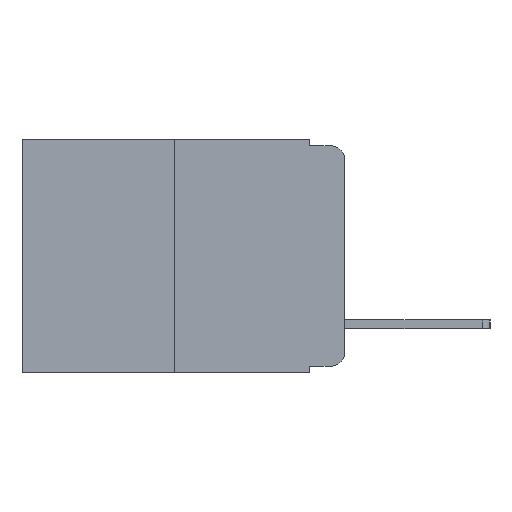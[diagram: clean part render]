
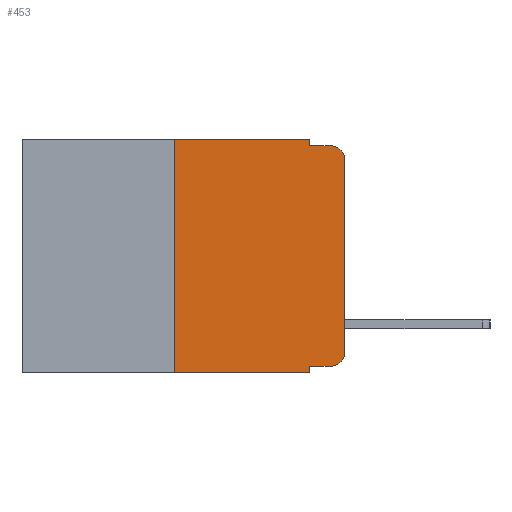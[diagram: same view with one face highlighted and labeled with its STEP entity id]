
A CAD part, left-side view. The second image highlights one B-rep face of the part: STEP entity #453.
In plain terms, the highlighted planar face has unit normal (-1, 0, 0).
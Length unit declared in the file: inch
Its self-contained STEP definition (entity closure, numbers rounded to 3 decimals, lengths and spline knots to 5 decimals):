
#366 = DIRECTION ( 'NONE',  ( 0., 0., 1. ) ) ;
#453 = ADVANCED_FACE ( 'NONE', ( #6808 ), #9087, .F. ) ;
#992 = CARTESIAN_POINT ( 'NONE',  ( 0., 0.25, 0. ) ) ;
#1239 = VERTEX_POINT ( 'NONE', #10865 ) ;
#1423 = DIRECTION ( 'NONE',  ( 0., -1., 0. ) ) ;
#1440 = CARTESIAN_POINT ( 'NONE',  ( 0., 0.051, 0. ) ) ;
#1443 = CARTESIAN_POINT ( 'NONE',  ( 0., 0., 0. ) ) ;
#1495 = VERTEX_POINT ( 'NONE', #3491 ) ;
#1644 = VECTOR ( 'NONE', #8561, 39.37008 ) ;
#1826 = CARTESIAN_POINT ( 'NONE',  ( 0., 0.051, -0.333 ) ) ;
#2103 = VERTEX_POINT ( 'NONE', #5677 ) ;
#2142 = VECTOR ( 'NONE', #11102, 39.37008 ) ;
#2264 = CARTESIAN_POINT ( 'NONE',  ( 0., 0.051, -0.01 ) ) ;
#2423 = VECTOR ( 'NONE', #1423, 39.37008 ) ;
#2447 = DIRECTION ( 'NONE',  ( 0., 0., -1. ) ) ;
#2634 = CARTESIAN_POINT ( 'NONE',  ( 0., 0.02, -0.333 ) ) ;
#2748 = AXIS2_PLACEMENT_3D ( 'NONE', #5929, #4686, #7265 ) ;
#3491 = CARTESIAN_POINT ( 'NONE',  ( 0., 0.051, -0.333 ) ) ;
#3553 = ORIENTED_EDGE ( 'NONE', *, *, #5797, .T. ) ;
#3752 = ORIENTED_EDGE ( 'NONE', *, *, #7470, .T. ) ;
#3794 = EDGE_CURVE ( 'NONE', #7345, #9619, #9673, .T. ) ;
#4267 = EDGE_CURVE ( 'NONE', #9619, #1239, #7231, .T. ) ;
#4373 = LINE ( 'NONE', #9382, #1644 ) ;
#4440 = EDGE_LOOP ( 'NONE', ( #3553, #3752, #4926, #5166, #5192, #5324, #5936, #6042, #6184, #6228 ) ) ;
#4561 = CARTESIAN_POINT ( 'NONE',  ( 0., 0.25, 0. ) ) ;
#4566 = DIRECTION ( 'NONE',  ( -1., 0., 0. ) ) ;
#4616 = CARTESIAN_POINT ( 'NONE',  ( 0., 0.02, -0.313 ) ) ;
#4645 = CIRCLE ( 'NONE', #5141, 0.02 ) ;
#4686 = DIRECTION ( 'NONE',  ( 1., 0., 0. ) ) ;
#4806 = LINE ( 'NONE', #1826, #2142 ) ;
#4926 = ORIENTED_EDGE ( 'NONE', *, *, #4267, .F. ) ;
#4931 = CARTESIAN_POINT ( 'NONE',  ( 0., 0.473, 0. ) ) ;
#5083 = VERTEX_POINT ( 'NONE', #10128 ) ;
#5141 = AXIS2_PLACEMENT_3D ( 'NONE', #9532, #4566, #10337 ) ;
#5163 = VERTEX_POINT ( 'NONE', #2634 ) ;
#5166 = ORIENTED_EDGE ( 'NONE', *, *, #3794, .F. ) ;
#5192 = ORIENTED_EDGE ( 'NONE', *, *, #10525, .F. ) ;
#5279 = VECTOR ( 'NONE', #2447, 39.37008 ) ;
#5324 = ORIENTED_EDGE ( 'NONE', *, *, #8269, .F. ) ;
#5353 = VERTEX_POINT ( 'NONE', #8778 ) ;
#5475 = DIRECTION ( 'NONE',  ( 0., 0., -1. ) ) ;
#5612 = LINE ( 'NONE', #1443, #9738 ) ;
#5677 = CARTESIAN_POINT ( 'NONE',  ( 0., 0.051, -0.343 ) ) ;
#5797 = EDGE_CURVE ( 'NONE', #5353, #8153, #5612, .T. ) ;
#5929 = CARTESIAN_POINT ( 'NONE',  ( 0., 0.473, 0. ) ) ;
#5936 = ORIENTED_EDGE ( 'NONE', *, *, #7177, .T. ) ;
#5962 = CIRCLE ( 'NONE', #7785, 0.02 ) ;
#6042 = ORIENTED_EDGE ( 'NONE', *, *, #8030, .F. ) ;
#6184 = ORIENTED_EDGE ( 'NONE', *, *, #6279, .T. ) ;
#6228 = ORIENTED_EDGE ( 'NONE', *, *, #6751, .T. ) ;
#6279 = EDGE_CURVE ( 'NONE', #1495, #5163, #4806, .T. ) ;
#6413 = CARTESIAN_POINT ( 'NONE',  ( 0., 0.051, -0.01 ) ) ;
#6751 = EDGE_CURVE ( 'NONE', #5163, #5353, #5962, .T. ) ;
#6808 = FACE_OUTER_BOUND ( 'NONE', #4440, .T. ) ;
#7177 = EDGE_CURVE ( 'NONE', #5083, #2103, #9196, .T. ) ;
#7231 = LINE ( 'NONE', #2264, #9156 ) ;
#7265 = DIRECTION ( 'NONE',  ( 0., 0., -1. ) ) ;
#7345 = VERTEX_POINT ( 'NONE', #10946 ) ;
#7425 = DIRECTION ( 'NONE',  ( 0., -1., 0. ) ) ;
#7470 = EDGE_CURVE ( 'NONE', #8153, #1239, #4645, .T. ) ;
#7602 = VECTOR ( 'NONE', #8293, 39.37008 ) ;
#7785 = AXIS2_PLACEMENT_3D ( 'NONE', #4616, #10384, #5475 ) ;
#7883 = VECTOR ( 'NONE', #8879, 39.37008 ) ;
#8030 = EDGE_CURVE ( 'NONE', #1495, #2103, #4373, .T. ) ;
#8153 = VERTEX_POINT ( 'NONE', #8735 ) ;
#8269 = EDGE_CURVE ( 'NONE', #5083, #10881, #10052, .T. ) ;
#8293 = DIRECTION ( 'NONE',  ( 0., -1., 0. ) ) ;
#8561 = DIRECTION ( 'NONE',  ( 0., 0., -1. ) ) ;
#8735 = CARTESIAN_POINT ( 'NONE',  ( 0., 0., -0.03 ) ) ;
#8778 = CARTESIAN_POINT ( 'NONE',  ( 0., 0., -0.313 ) ) ;
#8879 = DIRECTION ( 'NONE',  ( 0., 0., 1. ) ) ;
#9087 = PLANE ( 'NONE',  #2748 ) ;
#9156 = VECTOR ( 'NONE', #7425, 39.37008 ) ;
#9196 = LINE ( 'NONE', #9215, #2423 ) ;
#9215 = CARTESIAN_POINT ( 'NONE',  ( 0., 0.473, -0.343 ) ) ;
#9382 = CARTESIAN_POINT ( 'NONE',  ( 0., 0.051, 0. ) ) ;
#9532 = CARTESIAN_POINT ( 'NONE',  ( 0., 0.02, -0.03 ) ) ;
#9619 = VERTEX_POINT ( 'NONE', #6413 ) ;
#9673 = LINE ( 'NONE', #1440, #5279 ) ;
#9738 = VECTOR ( 'NONE', #366, 39.37008 ) ;
#9782 = LINE ( 'NONE', #4931, #7602 ) ;
#10052 = LINE ( 'NONE', #992, #7883 ) ;
#10128 = CARTESIAN_POINT ( 'NONE',  ( 0., 0.25, -0.343 ) ) ;
#10337 = DIRECTION ( 'NONE',  ( 0., 0., -1. ) ) ;
#10384 = DIRECTION ( 'NONE',  ( -1., 0., 0. ) ) ;
#10525 = EDGE_CURVE ( 'NONE', #10881, #7345, #9782, .T. ) ;
#10865 = CARTESIAN_POINT ( 'NONE',  ( 0., 0.02, -0.01 ) ) ;
#10881 = VERTEX_POINT ( 'NONE', #4561 ) ;
#10946 = CARTESIAN_POINT ( 'NONE',  ( 0., 0.051, 0. ) ) ;
#11102 = DIRECTION ( 'NONE',  ( 0., -1., 0. ) ) ;
